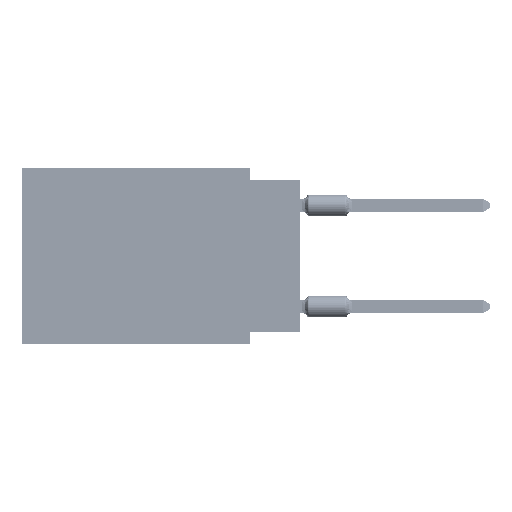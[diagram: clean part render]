
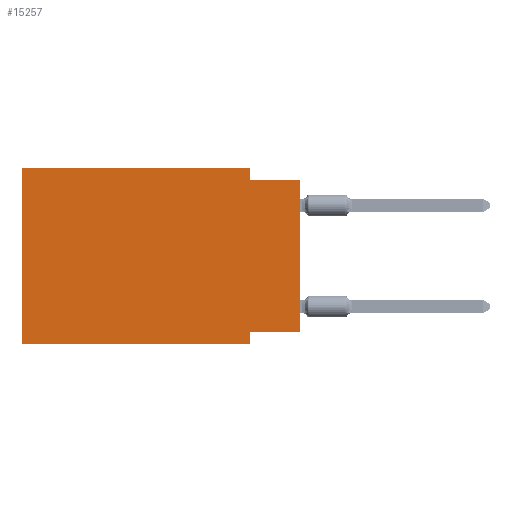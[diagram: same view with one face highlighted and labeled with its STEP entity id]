
A CAD part, left-side view. The second image highlights one B-rep face of the part: STEP entity #15257.
In plain terms, the highlighted planar face has unit normal (-1, 0, 0).
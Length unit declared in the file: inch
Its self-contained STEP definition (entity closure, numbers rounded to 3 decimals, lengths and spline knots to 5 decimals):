
#555 = ORIENTED_EDGE ( 'NONE', *, *, #50072, .F. ) ;
#650 = VECTOR ( 'NONE', #13770, 39.37008 ) ;
#819 = VERTEX_POINT ( 'NONE', #82097 ) ;
#1304 = CARTESIAN_POINT ( 'NONE',  ( 0., 0.55, -0.35 ) ) ;
#1684 = LINE ( 'NONE', #59386, #79046 ) ;
#2350 = EDGE_CURVE ( 'NONE', #33519, #819, #64498, .T. ) ;
#2365 = DIRECTION ( 'NONE',  ( 0., -1., 0. ) ) ;
#3091 = EDGE_LOOP ( 'NONE', ( #31624, #555, #58887, #61449, #11605, #13484, #25792, #65835 ) ) ;
#10317 = LINE ( 'NONE', #1304, #94760 ) ;
#11605 = ORIENTED_EDGE ( 'NONE', *, *, #73855, .F. ) ;
#12320 = DIRECTION ( 'NONE',  ( 0., 0., 1. ) ) ;
#13020 = VECTOR ( 'NONE', #98722, 39.37008 ) ;
#13484 = ORIENTED_EDGE ( 'NONE', *, *, #42325, .T. ) ;
#13770 = DIRECTION ( 'NONE',  ( 0., -1., 0. ) ) ;
#14725 = DIRECTION ( 'NONE',  ( 0., 1., 0. ) ) ;
#15257 = ADVANCED_FACE ( 'NONE', ( #25661 ), #58482, .F. ) ;
#19541 = VECTOR ( 'NONE', #14725, 39.37008 ) ;
#19868 = EDGE_CURVE ( 'NONE', #101071, #65956, #51931, .T. ) ;
#21789 = CARTESIAN_POINT ( 'NONE',  ( 0., 0.55, 0. ) ) ;
#25661 = FACE_OUTER_BOUND ( 'NONE', #3091, .T. ) ;
#25792 = ORIENTED_EDGE ( 'NONE', *, *, #73260, .F. ) ;
#27244 = CARTESIAN_POINT ( 'NONE',  ( 0., 0.55, 0. ) ) ;
#27282 = VERTEX_POINT ( 'NONE', #93490 ) ;
#27591 = CARTESIAN_POINT ( 'NONE',  ( 0., 0., -0.325 ) ) ;
#28631 = CARTESIAN_POINT ( 'NONE',  ( 0., 0.55, 0. ) ) ;
#28743 = CARTESIAN_POINT ( 'NONE',  ( 0., 0., 0. ) ) ;
#29219 = CARTESIAN_POINT ( 'NONE',  ( 0., 0., -0.025 ) ) ;
#31046 = LINE ( 'NONE', #55378, #82030 ) ;
#31624 = ORIENTED_EDGE ( 'NONE', *, *, #104665, .T. ) ;
#33519 = VERTEX_POINT ( 'NONE', #27591 ) ;
#34122 = CARTESIAN_POINT ( 'NONE',  ( 0., 0.1, -0.35 ) ) ;
#34153 = DIRECTION ( 'NONE',  ( 1., 0., 0. ) ) ;
#37952 = DIRECTION ( 'NONE',  ( 0., 0., -1. ) ) ;
#39462 = VECTOR ( 'NONE', #61504, 39.37008 ) ;
#39962 = LINE ( 'NONE', #34122, #13020 ) ;
#40479 = VECTOR ( 'NONE', #12320, 39.37008 ) ;
#42325 = EDGE_CURVE ( 'NONE', #102634, #27282, #10317, .T. ) ;
#44974 = VERTEX_POINT ( 'NONE', #68784 ) ;
#45649 = AXIS2_PLACEMENT_3D ( 'NONE', #27244, #34153, #90831 ) ;
#50072 = EDGE_CURVE ( 'NONE', #78196, #44974, #101790, .T. ) ;
#51931 = LINE ( 'NONE', #28631, #650 ) ;
#53850 = CARTESIAN_POINT ( 'NONE',  ( 0., 0.1, -0.025 ) ) ;
#55378 = CARTESIAN_POINT ( 'NONE',  ( 0., 0.1, 0. ) ) ;
#56722 = CARTESIAN_POINT ( 'NONE',  ( 0., 0.1, 0. ) ) ;
#58482 = PLANE ( 'NONE',  #45649 ) ;
#58887 = ORIENTED_EDGE ( 'NONE', *, *, #95835, .F. ) ;
#59386 = CARTESIAN_POINT ( 'NONE',  ( 0., 0.55, 0. ) ) ;
#61449 = ORIENTED_EDGE ( 'NONE', *, *, #19868, .F. ) ;
#61504 = DIRECTION ( 'NONE',  ( 0., -1., 0. ) ) ;
#64498 = LINE ( 'NONE', #72958, #19541 ) ;
#65835 = ORIENTED_EDGE ( 'NONE', *, *, #2350, .F. ) ;
#65956 = VERTEX_POINT ( 'NONE', #56722 ) ;
#67849 = DIRECTION ( 'NONE',  ( 0., 0., 1. ) ) ;
#68784 = CARTESIAN_POINT ( 'NONE',  ( 0., 0., -0.025 ) ) ;
#72958 = CARTESIAN_POINT ( 'NONE',  ( 0., 0., -0.325 ) ) ;
#73260 = EDGE_CURVE ( 'NONE', #819, #27282, #39962, .T. ) ;
#73855 = EDGE_CURVE ( 'NONE', #102634, #101071, #1684, .T. ) ;
#78196 = VERTEX_POINT ( 'NONE', #53850 ) ;
#79046 = VECTOR ( 'NONE', #67849, 39.37008 ) ;
#82030 = VECTOR ( 'NONE', #37952, 39.37008 ) ;
#82097 = CARTESIAN_POINT ( 'NONE',  ( 0., 0.1, -0.325 ) ) ;
#90831 = DIRECTION ( 'NONE',  ( 0., 0., -1. ) ) ;
#93490 = CARTESIAN_POINT ( 'NONE',  ( 0., 0.1, -0.35 ) ) ;
#94760 = VECTOR ( 'NONE', #2365, 39.37008 ) ;
#95278 = CARTESIAN_POINT ( 'NONE',  ( 0., 0.55, -0.35 ) ) ;
#95835 = EDGE_CURVE ( 'NONE', #65956, #78196, #31046, .T. ) ;
#98722 = DIRECTION ( 'NONE',  ( 0., 0., -1. ) ) ;
#101071 = VERTEX_POINT ( 'NONE', #21789 ) ;
#101304 = LINE ( 'NONE', #28743, #40479 ) ;
#101790 = LINE ( 'NONE', #29219, #39462 ) ;
#102634 = VERTEX_POINT ( 'NONE', #95278 ) ;
#104665 = EDGE_CURVE ( 'NONE', #33519, #44974, #101304, .T. ) ;
